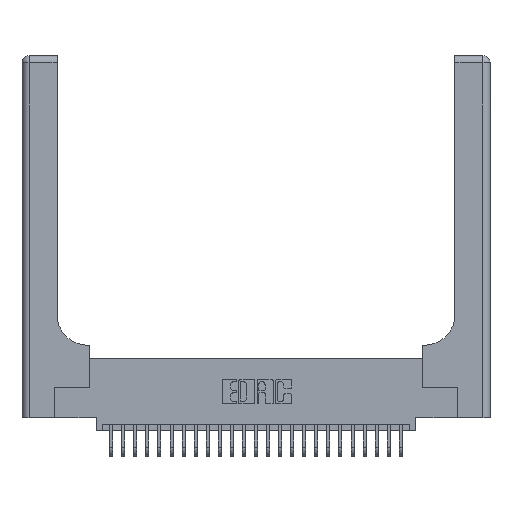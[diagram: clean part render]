
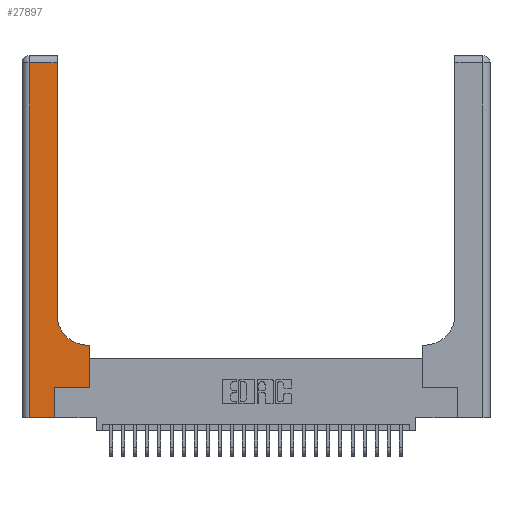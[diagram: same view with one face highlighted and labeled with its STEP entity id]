
A CAD part, top view. The second image highlights one B-rep face of the part: STEP entity #27897.
In plain terms, the highlighted planar face has unit normal (0, 0, 1).
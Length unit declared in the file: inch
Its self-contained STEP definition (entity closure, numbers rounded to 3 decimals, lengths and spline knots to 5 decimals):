
#453 = VERTEX_POINT ( 'NONE', #15389 ) ;
#498 = LINE ( 'NONE', #3648, #4668 ) ;
#837 = CARTESIAN_POINT ( 'NONE',  ( 0., 2.94, 0.37 ) ) ;
#2110 = DIRECTION ( 'NONE',  ( 0., 1., 0. ) ) ;
#2572 = EDGE_LOOP ( 'NONE', ( #24874, #11851, #26896, #27032, #4346, #15545, #8083, #6301, #24695 ) ) ;
#2763 = LINE ( 'NONE', #17249, #19791 ) ;
#3306 = EDGE_CURVE ( 'NONE', #21721, #22265, #8102, .T. ) ;
#3606 = CARTESIAN_POINT ( 'NONE',  ( 0., 0., 0.37 ) ) ;
#3648 = CARTESIAN_POINT ( 'NONE',  ( 0.2915, 0.6, 0.37 ) ) ;
#4346 = ORIENTED_EDGE ( 'NONE', *, *, #20019, .T. ) ;
#4618 = VECTOR ( 'NONE', #19780, 39.37008 ) ;
#4668 = VECTOR ( 'NONE', #19189, 39.37008 ) ;
#5173 = VERTEX_POINT ( 'NONE', #26547 ) ;
#5429 = DIRECTION ( 'NONE',  ( 1., 0., 0. ) ) ;
#5637 = EDGE_CURVE ( 'NONE', #453, #16365, #2763, .T. ) ;
#5856 = PLANE ( 'NONE',  #8064 ) ;
#5883 = DIRECTION ( 'NONE',  ( 1., 0., 0. ) ) ;
#6301 = ORIENTED_EDGE ( 'NONE', *, *, #7476, .T. ) ;
#6606 = CARTESIAN_POINT ( 'NONE',  ( 0.5585, 0.25, 0.37 ) ) ;
#6737 = LINE ( 'NONE', #3606, #27689 ) ;
#7476 = EDGE_CURVE ( 'NONE', #5173, #27816, #498, .T. ) ;
#8064 = AXIS2_PLACEMENT_3D ( 'NONE', #10613, #15051, #25927 ) ;
#8083 = ORIENTED_EDGE ( 'NONE', *, *, #19866, .T. ) ;
#8102 = LINE ( 'NONE', #8593, #4618 ) ;
#8111 = CARTESIAN_POINT ( 'NONE',  ( 0.2915, 2.94, 0.37 ) ) ;
#8217 = VECTOR ( 'NONE', #2110, 39.37008 ) ;
#8593 = CARTESIAN_POINT ( 'NONE',  ( 0.06, 3., 0.37 ) ) ;
#8785 = VERTEX_POINT ( 'NONE', #15652 ) ;
#10613 = CARTESIAN_POINT ( 'NONE',  ( 0., 3., 0.37 ) ) ;
#10774 = CARTESIAN_POINT ( 'NONE',  ( 0.269, 0., 0.37 ) ) ;
#11073 = CARTESIAN_POINT ( 'NONE',  ( 0.5415, 0.85, 0.37 ) ) ;
#11078 = CARTESIAN_POINT ( 'NONE',  ( 0.5585, 0.25, 0.37 ) ) ;
#11851 = ORIENTED_EDGE ( 'NONE', *, *, #17223, .T. ) ;
#12197 = VECTOR ( 'NONE', #12461, 39.37008 ) ;
#12461 = DIRECTION ( 'NONE',  ( 0., 1., 0. ) ) ;
#12469 = DIRECTION ( 'NONE',  ( 1., 0., 0. ) ) ;
#12759 = CARTESIAN_POINT ( 'NONE',  ( 0.5415, 0.6, 0.37 ) ) ;
#15051 = DIRECTION ( 'NONE',  ( 0., 0., -1. ) ) ;
#15389 = CARTESIAN_POINT ( 'NONE',  ( 0.269, 0.25, 0.37 ) ) ;
#15545 = ORIENTED_EDGE ( 'NONE', *, *, #5637, .T. ) ;
#15614 = CIRCLE ( 'NONE', #28202, 0.25 ) ;
#15652 = CARTESIAN_POINT ( 'NONE',  ( 0.2915, 0.85, 0.37 ) ) ;
#16211 = VECTOR ( 'NONE', #27486, 39.37008 ) ;
#16365 = VERTEX_POINT ( 'NONE', #6606 ) ;
#17223 = EDGE_CURVE ( 'NONE', #22863, #21721, #19336, .T. ) ;
#17249 = CARTESIAN_POINT ( 'NONE',  ( 0.269, 0.25, 0.37 ) ) ;
#17937 = LINE ( 'NONE', #23068, #16211 ) ;
#19189 = DIRECTION ( 'NONE',  ( -1., 0., 0. ) ) ;
#19336 = LINE ( 'NONE', #837, #21780 ) ;
#19780 = DIRECTION ( 'NONE',  ( 0., -1., 0. ) ) ;
#19791 = VECTOR ( 'NONE', #5883, 39.37008 ) ;
#19866 = EDGE_CURVE ( 'NONE', #16365, #5173, #25999, .T. ) ;
#20019 = EDGE_CURVE ( 'NONE', #24227, #453, #17937, .T. ) ;
#21395 = EDGE_CURVE ( 'NONE', #22265, #24227, #6737, .T. ) ;
#21721 = VERTEX_POINT ( 'NONE', #24259 ) ;
#21780 = VECTOR ( 'NONE', #25377, 39.37008 ) ;
#22265 = VERTEX_POINT ( 'NONE', #28642 ) ;
#22863 = VERTEX_POINT ( 'NONE', #8111 ) ;
#23068 = CARTESIAN_POINT ( 'NONE',  ( 0.269, 0., 0.37 ) ) ;
#23264 = DIRECTION ( 'NONE',  ( 0., 0., -1. ) ) ;
#23592 = EDGE_CURVE ( 'NONE', #8785, #22863, #24381, .T. ) ;
#23838 = EDGE_CURVE ( 'NONE', #27816, #8785, #15614, .T. ) ;
#24227 = VERTEX_POINT ( 'NONE', #10774 ) ;
#24259 = CARTESIAN_POINT ( 'NONE',  ( 0.06, 2.94, 0.37 ) ) ;
#24381 = LINE ( 'NONE', #25822, #12197 ) ;
#24695 = ORIENTED_EDGE ( 'NONE', *, *, #23838, .T. ) ;
#24874 = ORIENTED_EDGE ( 'NONE', *, *, #23592, .T. ) ;
#25377 = DIRECTION ( 'NONE',  ( -1., 0., 0. ) ) ;
#25822 = CARTESIAN_POINT ( 'NONE',  ( 0.2915, 3., 0.37 ) ) ;
#25927 = DIRECTION ( 'NONE',  ( -1., 0., 0. ) ) ;
#25999 = LINE ( 'NONE', #11078, #8217 ) ;
#26547 = CARTESIAN_POINT ( 'NONE',  ( 0.5585, 0.6, 0.37 ) ) ;
#26896 = ORIENTED_EDGE ( 'NONE', *, *, #3306, .T. ) ;
#27032 = ORIENTED_EDGE ( 'NONE', *, *, #21395, .T. ) ;
#27453 = FACE_OUTER_BOUND ( 'NONE', #2572, .T. ) ;
#27486 = DIRECTION ( 'NONE',  ( 0., 1., 0. ) ) ;
#27689 = VECTOR ( 'NONE', #12469, 39.37008 ) ;
#27816 = VERTEX_POINT ( 'NONE', #12759 ) ;
#27897 = ADVANCED_FACE ( 'NONE', ( #27453 ), #5856, .F. ) ;
#28202 = AXIS2_PLACEMENT_3D ( 'NONE', #11073, #23264, #5429 ) ;
#28642 = CARTESIAN_POINT ( 'NONE',  ( 0.06, 0., 0.37 ) ) ;
